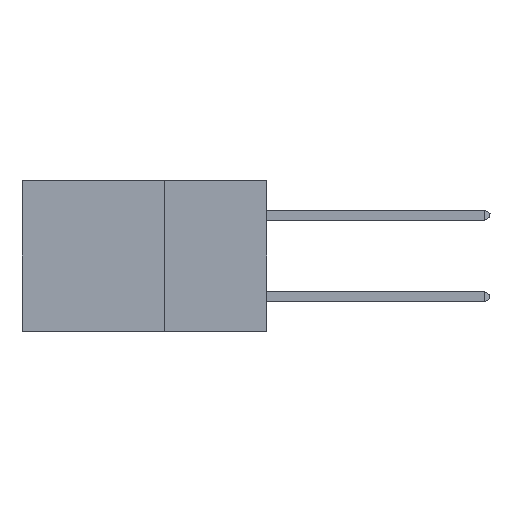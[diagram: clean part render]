
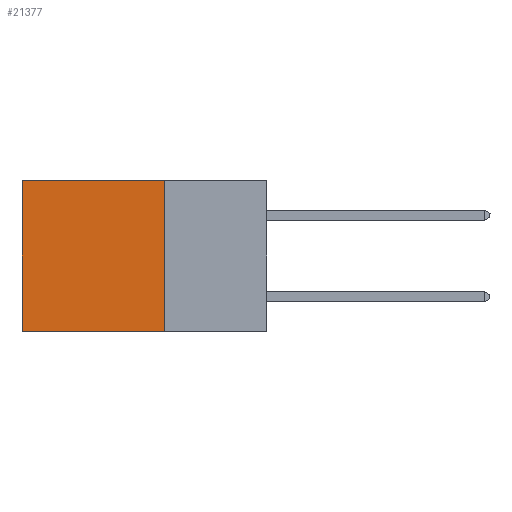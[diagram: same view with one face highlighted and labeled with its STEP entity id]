
A CAD part, left-side view. The second image highlights one B-rep face of the part: STEP entity #21377.
In plain terms, the highlighted planar face has unit normal (-1, 0, 0).
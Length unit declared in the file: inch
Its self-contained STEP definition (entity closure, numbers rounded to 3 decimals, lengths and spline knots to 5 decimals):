
#236 = ORIENTED_EDGE ( 'NONE', *, *, #4000, .T. ) ;
#1022 = CARTESIAN_POINT ( 'NONE',  ( 0.2875, 0.25, 0. ) ) ;
#1419 = DIRECTION ( 'NONE',  ( 0., 0., -1. ) ) ;
#1945 = DIRECTION ( 'NONE',  ( 0., 1., 0. ) ) ;
#3180 = VERTEX_POINT ( 'NONE', #21370 ) ;
#3291 = EDGE_CURVE ( 'NONE', #5617, #14210, #12874, .T. ) ;
#3628 = PLANE ( 'NONE',  #4077 ) ;
#4000 = EDGE_CURVE ( 'NONE', #5617, #3180, #15576, .T. ) ;
#4077 = AXIS2_PLACEMENT_3D ( 'NONE', #11290, #11162, #13096 ) ;
#5290 = LINE ( 'NONE', #5419, #6859 ) ;
#5419 = CARTESIAN_POINT ( 'NONE',  ( 0.2875, 0.6, 0. ) ) ;
#5617 = VERTEX_POINT ( 'NONE', #1022 ) ;
#6491 = DIRECTION ( 'NONE',  ( 0., 0., -1. ) ) ;
#6859 = VECTOR ( 'NONE', #1419, 39.37008 ) ;
#7265 = EDGE_CURVE ( 'NONE', #3180, #14870, #5290, .T. ) ;
#7798 = CARTESIAN_POINT ( 'NONE',  ( 0.2875, 0.25, -0.37 ) ) ;
#11162 = DIRECTION ( 'NONE',  ( 1., 0., 0. ) ) ;
#11290 = CARTESIAN_POINT ( 'NONE',  ( 0.2875, 0.25, 0. ) ) ;
#11614 = EDGE_CURVE ( 'NONE', #14210, #14870, #19362, .T. ) ;
#12759 = ORIENTED_EDGE ( 'NONE', *, *, #11614, .F. ) ;
#12874 = LINE ( 'NONE', #24536, #14677 ) ;
#13096 = DIRECTION ( 'NONE',  ( 0., 0., -1. ) ) ;
#14210 = VERTEX_POINT ( 'NONE', #7798 ) ;
#14677 = VECTOR ( 'NONE', #6491, 39.37008 ) ;
#14870 = VERTEX_POINT ( 'NONE', #19060 ) ;
#15129 = ORIENTED_EDGE ( 'NONE', *, *, #3291, .F. ) ;
#15187 = FACE_OUTER_BOUND ( 'NONE', #15718, .T. ) ;
#15576 = LINE ( 'NONE', #19854, #24927 ) ;
#15718 = EDGE_LOOP ( 'NONE', ( #18248, #12759, #15129, #236 ) ) ;
#18248 = ORIENTED_EDGE ( 'NONE', *, *, #7265, .T. ) ;
#19060 = CARTESIAN_POINT ( 'NONE',  ( 0.2875, 0.6, -0.37 ) ) ;
#19362 = LINE ( 'NONE', #21558, #24866 ) ;
#19854 = CARTESIAN_POINT ( 'NONE',  ( 0.2875, 0.25, 0. ) ) ;
#21370 = CARTESIAN_POINT ( 'NONE',  ( 0.2875, 0.6, 0. ) ) ;
#21377 = ADVANCED_FACE ( 'NONE', ( #15187 ), #3628, .F. ) ;
#21558 = CARTESIAN_POINT ( 'NONE',  ( 0.2875, 0.25, -0.37 ) ) ;
#24536 = CARTESIAN_POINT ( 'NONE',  ( 0.2875, 0.25, 0. ) ) ;
#24866 = VECTOR ( 'NONE', #1945, 39.37008 ) ;
#24927 = VECTOR ( 'NONE', #25530, 39.37008 ) ;
#25530 = DIRECTION ( 'NONE',  ( 0., 1., 0. ) ) ;
